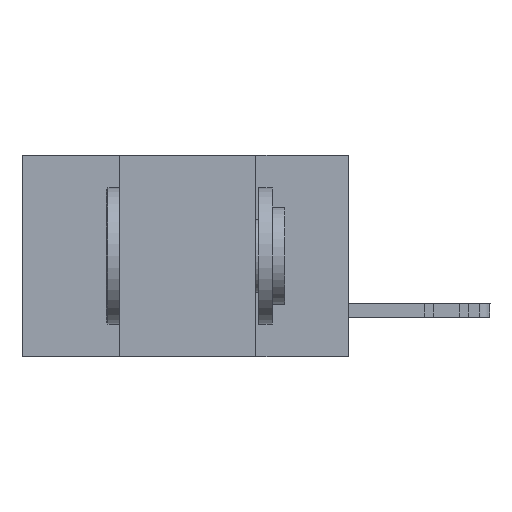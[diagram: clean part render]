
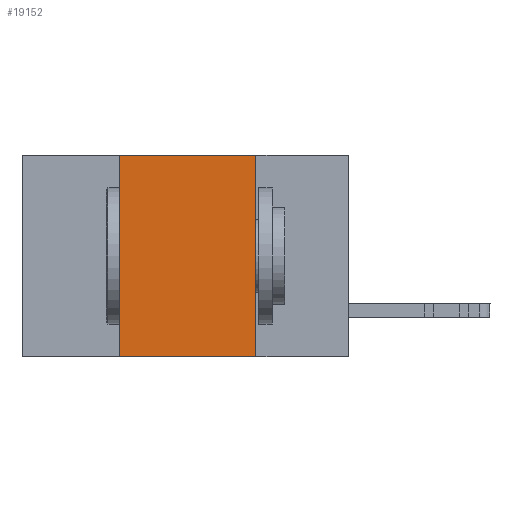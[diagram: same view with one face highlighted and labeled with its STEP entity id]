
A CAD part, left-side view. The second image highlights one B-rep face of the part: STEP entity #19152.
In plain terms, the highlighted planar face has unit normal (-1, 0, 0).
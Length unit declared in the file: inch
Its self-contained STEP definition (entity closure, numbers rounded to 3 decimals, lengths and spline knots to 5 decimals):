
#494 = ORIENTED_EDGE ( 'NONE', *, *, #16928, .T. ) ;
#1865 = VECTOR ( 'NONE', #5103, 39.37008 ) ;
#2198 = DIRECTION ( 'NONE',  ( 0., 0., 1. ) ) ;
#2448 = VERTEX_POINT ( 'NONE', #7885 ) ;
#3252 = CARTESIAN_POINT ( 'NONE',  ( 0., 0.6, -0.37 ) ) ;
#3432 = LINE ( 'NONE', #8977, #12664 ) ;
#4058 = VERTEX_POINT ( 'NONE', #4615 ) ;
#4525 = EDGE_CURVE ( 'NONE', #2448, #4058, #3432, .T. ) ;
#4615 = CARTESIAN_POINT ( 'NONE',  ( 0., 0.17, 0. ) ) ;
#4675 = FACE_OUTER_BOUND ( 'NONE', #18142, .T. ) ;
#5101 = VECTOR ( 'NONE', #16271, 39.37008 ) ;
#5103 = DIRECTION ( 'NONE',  ( 0., -1., 0. ) ) ;
#5646 = VECTOR ( 'NONE', #2198, 39.37008 ) ;
#6888 = ORIENTED_EDGE ( 'NONE', *, *, #15715, .F. ) ;
#7456 = ORIENTED_EDGE ( 'NONE', *, *, #4525, .F. ) ;
#7885 = CARTESIAN_POINT ( 'NONE',  ( 0., 0.42, 0. ) ) ;
#8551 = AXIS2_PLACEMENT_3D ( 'NONE', #9680, #22304, #11579 ) ;
#8571 = DIRECTION ( 'NONE',  ( 0., -1., 0. ) ) ;
#8977 = CARTESIAN_POINT ( 'NONE',  ( 0., 0.6, 0. ) ) ;
#9680 = CARTESIAN_POINT ( 'NONE',  ( 0., 0.6, 0. ) ) ;
#11579 = DIRECTION ( 'NONE',  ( 0., 0., -1. ) ) ;
#11690 = LINE ( 'NONE', #3252, #1865 ) ;
#12664 = VECTOR ( 'NONE', #8571, 39.37008 ) ;
#13004 = CARTESIAN_POINT ( 'NONE',  ( 0., 0.42, -0.37 ) ) ;
#13216 = CARTESIAN_POINT ( 'NONE',  ( 0., 0.42, -0.37 ) ) ;
#13600 = ORIENTED_EDGE ( 'NONE', *, *, #23125, .F. ) ;
#14426 = CARTESIAN_POINT ( 'NONE',  ( 0., 0.17, -0.37 ) ) ;
#14998 = LINE ( 'NONE', #14426, #5101 ) ;
#15503 = LINE ( 'NONE', #13216, #5646 ) ;
#15715 = EDGE_CURVE ( 'NONE', #4058, #22529, #14998, .T. ) ;
#16271 = DIRECTION ( 'NONE',  ( 0., 0., -1. ) ) ;
#16928 = EDGE_CURVE ( 'NONE', #22488, #22529, #11690, .T. ) ;
#18142 = EDGE_LOOP ( 'NONE', ( #6888, #7456, #13600, #494 ) ) ;
#18562 = CARTESIAN_POINT ( 'NONE',  ( 0., 0.17, -0.37 ) ) ;
#19152 = ADVANCED_FACE ( 'NONE', ( #4675 ), #21937, .F. ) ;
#21937 = PLANE ( 'NONE',  #8551 ) ;
#22304 = DIRECTION ( 'NONE',  ( 1., 0., 0. ) ) ;
#22488 = VERTEX_POINT ( 'NONE', #13004 ) ;
#22529 = VERTEX_POINT ( 'NONE', #18562 ) ;
#23125 = EDGE_CURVE ( 'NONE', #22488, #2448, #15503, .T. ) ;
